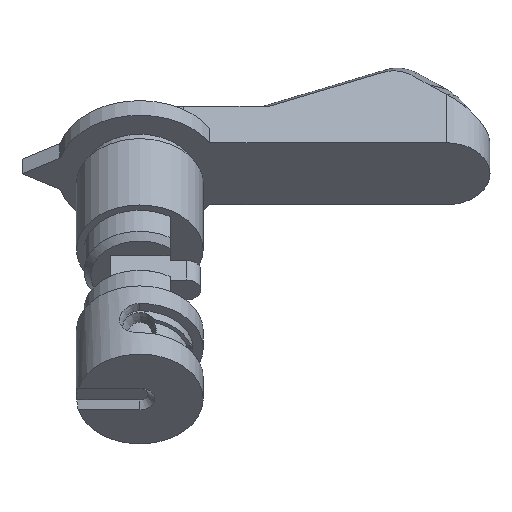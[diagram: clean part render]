
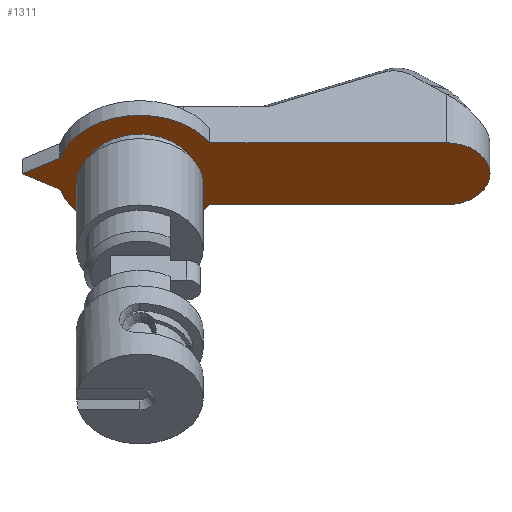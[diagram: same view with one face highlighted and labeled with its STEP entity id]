
A CAD part, front view. The second image highlights one B-rep face of the part: STEP entity #1311.
In plain terms, the highlighted planar face has unit normal (0, -0.707, -0.707).
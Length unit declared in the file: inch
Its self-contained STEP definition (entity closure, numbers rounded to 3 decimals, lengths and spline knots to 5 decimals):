
#31=FACE_BOUND('',#306,.T.);
#130=CIRCLE('',#1388,0.125);
#141=CIRCLE('',#1422,0.23622);
#143=CIRCLE('',#1425,0.23622);
#153=CIRCLE('',#1448,0.15945);
#231=FACE_OUTER_BOUND('',#305,.T.);
#305=EDGE_LOOP('',(#1180,#1181,#1182,#1183,#1184,#1185,#1186));
#306=EDGE_LOOP('',(#1187));
#347=LINE('',#1965,#440);
#372=LINE('',#2126,#465);
#389=LINE('',#2770,#482);
#393=LINE('',#2778,#486);
#440=VECTOR('',#1575,0.3937);
#465=VECTOR('',#1628,0.3937);
#482=VECTOR('',#1703,0.3937);
#486=VECTOR('',#1709,0.3937);
#562=VERTEX_POINT('',#1962);
#563=VERTEX_POINT('',#1964);
#578=VERTEX_POINT('',#2115);
#581=VERTEX_POINT('',#2124);
#618=VERTEX_POINT('',#2768);
#619=VERTEX_POINT('',#2769);
#622=VERTEX_POINT('',#2777);
#631=VERTEX_POINT('',#2825);
#700=EDGE_CURVE('',#562,#563,#347,.T.);
#729=EDGE_CURVE('',#578,#562,#130,.T.);
#733=EDGE_CURVE('',#581,#578,#372,.T.);
#792=EDGE_CURVE('',#618,#619,#389,.T.);
#796=EDGE_CURVE('',#622,#618,#393,.T.);
#799=EDGE_CURVE('',#563,#622,#141,.T.);
#801=EDGE_CURVE('',#619,#581,#143,.T.);
#820=EDGE_CURVE('',#631,#631,#153,.T.);
#1180=ORIENTED_EDGE('',*,*,#700,.F.);
#1181=ORIENTED_EDGE('',*,*,#729,.F.);
#1182=ORIENTED_EDGE('',*,*,#733,.F.);
#1183=ORIENTED_EDGE('',*,*,#801,.F.);
#1184=ORIENTED_EDGE('',*,*,#792,.F.);
#1185=ORIENTED_EDGE('',*,*,#796,.F.);
#1186=ORIENTED_EDGE('',*,*,#799,.F.);
#1187=ORIENTED_EDGE('',*,*,#820,.T.);
#1240=PLANE('',#1447);
#1311=ADVANCED_FACE('',(#231,#31),#1240,.F.);
#1388=AXIS2_PLACEMENT_3D('',#2117,#1619,#1620);
#1422=AXIS2_PLACEMENT_3D('',#2783,#1714,#1715);
#1425=AXIS2_PLACEMENT_3D('',#2786,#1720,#1721);
#1447=AXIS2_PLACEMENT_3D('',#2824,#1773,#1774);
#1448=AXIS2_PLACEMENT_3D('',#2826,#1775,#1776);
#1575=DIRECTION('',(-1.,0.,0.));
#1619=DIRECTION('center_axis',(0.,0.707,0.707));
#1620=DIRECTION('ref_axis',(0.,-0.707,0.707));
#1628=DIRECTION('',(1.,0.,0.));
#1703=DIRECTION('',(0.866,-0.354,0.354));
#1709=DIRECTION('',(-0.866,-0.354,0.354));
#1714=DIRECTION('center_axis',(0.,0.707,0.707));
#1715=DIRECTION('ref_axis',(1.,0.,0.));
#1720=DIRECTION('center_axis',(0.,0.707,0.707));
#1721=DIRECTION('ref_axis',(1.,0.,0.));
#1773=DIRECTION('center_axis',(0.,0.707,0.707));
#1774=DIRECTION('ref_axis',(1.,0.,0.));
#1775=DIRECTION('center_axis',(0.,0.707,0.707));
#1776=DIRECTION('ref_axis',(1.,0.,0.));
#1962=CARTESIAN_POINT('',(1.00886,0.21088,0.0341));
#1964=CARTESIAN_POINT('',(0.3343,0.21088,0.0341));
#1965=CARTESIAN_POINT('',(1.00886,0.21088,0.0341));
#2115=CARTESIAN_POINT('',(1.00886,0.0341,0.21088));
#2117=CARTESIAN_POINT('Origin',(1.00886,0.12249,0.12249));
#2124=CARTESIAN_POINT('',(0.3343,0.0341,0.21088));
#2126=CARTESIAN_POINT('',(0.25886,0.0341,0.21088));
#2768=CARTESIAN_POINT('',(-0.20236,0.12249,0.12249));
#2769=CARTESIAN_POINT('',(-0.09391,0.07822,0.16677));
#2770=CARTESIAN_POINT('',(-0.20236,0.12249,0.12249));
#2777=CARTESIAN_POINT('',(-0.09391,0.16677,0.07822));
#2778=CARTESIAN_POINT('',(-0.09391,0.16677,0.07822));
#2783=CARTESIAN_POINT('Origin',(0.13386,0.12249,0.12249));
#2786=CARTESIAN_POINT('Origin',(0.13386,0.12249,0.12249));
#2824=CARTESIAN_POINT('Origin',(0.63386,0.12249,0.12249));
#2825=CARTESIAN_POINT('',(-0.02559,0.12249,0.12249));
#2826=CARTESIAN_POINT('Origin',(0.13386,0.12249,0.12249));
